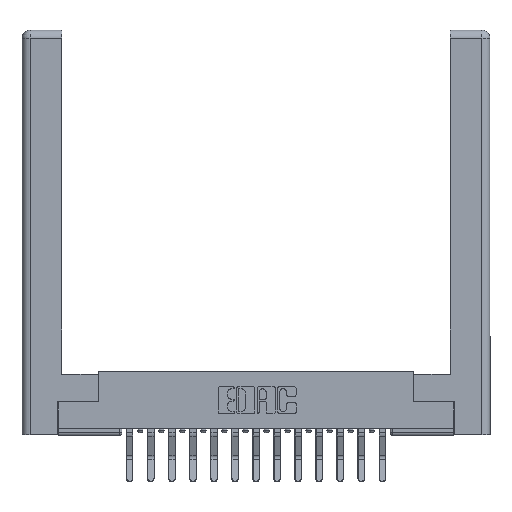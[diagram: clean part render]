
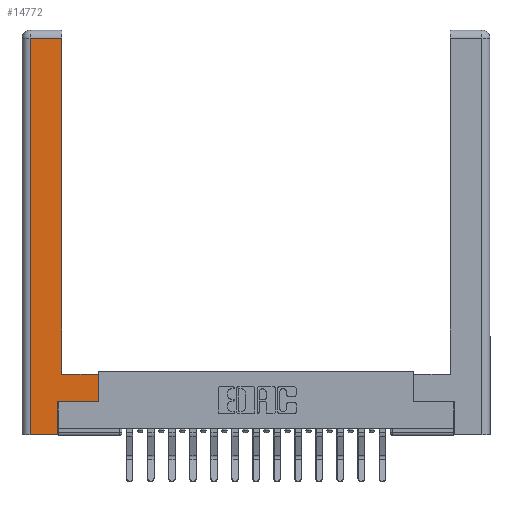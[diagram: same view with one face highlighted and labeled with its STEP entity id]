
A CAD part, top view. The second image highlights one B-rep face of the part: STEP entity #14772.
In plain terms, the highlighted planar face has unit normal (0, 0, 1).
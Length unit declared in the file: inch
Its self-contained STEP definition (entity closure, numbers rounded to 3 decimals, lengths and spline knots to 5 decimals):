
#153 = VECTOR ( 'NONE', #13332, 39.37008 ) ;
#187 = VERTEX_POINT ( 'NONE', #190 ) ;
#190 = CARTESIAN_POINT ( 'NONE',  ( 0.565, 0.245, 0. ) ) ;
#426 = DIRECTION ( 'NONE',  ( 0., 0., -1. ) ) ;
#797 = EDGE_LOOP ( 'NONE', ( #3934, #11235, #12973, #6935, #10437, #15343, #7932, #13033 ) ) ;
#1330 = DIRECTION ( 'NONE',  ( 1., 0., 0. ) ) ;
#1382 = LINE ( 'NONE', #16580, #14872 ) ;
#1908 = VECTOR ( 'NONE', #8428, 39.37008 ) ;
#1924 = VECTOR ( 'NONE', #4143, 39.37008 ) ;
#2317 = VERTEX_POINT ( 'NONE', #4496 ) ;
#2909 = CARTESIAN_POINT ( 'NONE',  ( 0.0615, 2.94, 0. ) ) ;
#2956 = EDGE_CURVE ( 'NONE', #187, #5258, #7629, .T. ) ;
#3008 = CARTESIAN_POINT ( 'NONE',  ( 0.565, 0.245, 0. ) ) ;
#3301 = EDGE_CURVE ( 'NONE', #8868, #14554, #16667, .T. ) ;
#3358 = EDGE_CURVE ( 'NONE', #13544, #8868, #1382, .T. ) ;
#3828 = CARTESIAN_POINT ( 'NONE',  ( 0.265, 0.245, 0. ) ) ;
#3934 = ORIENTED_EDGE ( 'NONE', *, *, #3358, .T. ) ;
#4034 = VECTOR ( 'NONE', #10311, 39.37008 ) ;
#4089 = VERTEX_POINT ( 'NONE', #16123 ) ;
#4143 = DIRECTION ( 'NONE',  ( 0., -1., 0. ) ) ;
#4176 = DIRECTION ( 'NONE',  ( 1., 0., 0. ) ) ;
#4496 = CARTESIAN_POINT ( 'NONE',  ( 0.0615, 0., 0. ) ) ;
#5122 = EDGE_CURVE ( 'NONE', #5258, #13544, #15570, .T. ) ;
#5258 = VERTEX_POINT ( 'NONE', #9324 ) ;
#5654 = LINE ( 'NONE', #17803, #12512 ) ;
#6290 = CARTESIAN_POINT ( 'NONE',  ( 0.295, 0.45, 0. ) ) ;
#6687 = VECTOR ( 'NONE', #10426, 39.37008 ) ;
#6935 = ORIENTED_EDGE ( 'NONE', *, *, #9998, .T. ) ;
#7108 = DIRECTION ( 'NONE',  ( -1., 0., 0. ) ) ;
#7629 = LINE ( 'NONE', #14586, #153 ) ;
#7859 = EDGE_CURVE ( 'NONE', #11265, #4089, #13507, .T. ) ;
#7932 = ORIENTED_EDGE ( 'NONE', *, *, #2956, .T. ) ;
#8428 = DIRECTION ( 'NONE',  ( -1., 0., 0. ) ) ;
#8730 = EDGE_CURVE ( 'NONE', #4089, #187, #11395, .T. ) ;
#8868 = VERTEX_POINT ( 'NONE', #11855 ) ;
#9324 = CARTESIAN_POINT ( 'NONE',  ( 0.565, 0.45, 0. ) ) ;
#9807 = CARTESIAN_POINT ( 'NONE',  ( 0., 0., 0. ) ) ;
#9998 = EDGE_CURVE ( 'NONE', #2317, #11265, #5654, .T. ) ;
#10311 = DIRECTION ( 'NONE',  ( -1., 0., 0. ) ) ;
#10426 = DIRECTION ( 'NONE',  ( 0., 1., 0. ) ) ;
#10437 = ORIENTED_EDGE ( 'NONE', *, *, #7859, .T. ) ;
#11059 = FACE_OUTER_BOUND ( 'NONE', #797, .T. ) ;
#11235 = ORIENTED_EDGE ( 'NONE', *, *, #3301, .T. ) ;
#11265 = VERTEX_POINT ( 'NONE', #14806 ) ;
#11395 = LINE ( 'NONE', #3008, #16839 ) ;
#11855 = CARTESIAN_POINT ( 'NONE',  ( 0.295, 2.94, 0. ) ) ;
#12023 = AXIS2_PLACEMENT_3D ( 'NONE', #9807, #426, #7108 ) ;
#12512 = VECTOR ( 'NONE', #1330, 39.37008 ) ;
#12689 = EDGE_CURVE ( 'NONE', #14554, #2317, #16370, .T. ) ;
#12973 = ORIENTED_EDGE ( 'NONE', *, *, #12689, .T. ) ;
#13033 = ORIENTED_EDGE ( 'NONE', *, *, #5122, .T. ) ;
#13332 = DIRECTION ( 'NONE',  ( 0., 1., 0. ) ) ;
#13507 = LINE ( 'NONE', #3828, #6687 ) ;
#13544 = VERTEX_POINT ( 'NONE', #6290 ) ;
#14554 = VERTEX_POINT ( 'NONE', #17897 ) ;
#14586 = CARTESIAN_POINT ( 'NONE',  ( 0.565, 0.45, 0. ) ) ;
#14772 = ADVANCED_FACE ( 'NONE', ( #11059 ), #16713, .F. ) ;
#14806 = CARTESIAN_POINT ( 'NONE',  ( 0.265, 0., 0. ) ) ;
#14813 = DIRECTION ( 'NONE',  ( 0., 1., 0. ) ) ;
#14872 = VECTOR ( 'NONE', #14813, 39.37008 ) ;
#15343 = ORIENTED_EDGE ( 'NONE', *, *, #8730, .T. ) ;
#15570 = LINE ( 'NONE', #17407, #4034 ) ;
#16123 = CARTESIAN_POINT ( 'NONE',  ( 0.265, 0.245, 0. ) ) ;
#16370 = LINE ( 'NONE', #17828, #1924 ) ;
#16580 = CARTESIAN_POINT ( 'NONE',  ( 0.295, 3., 0. ) ) ;
#16667 = LINE ( 'NONE', #2909, #1908 ) ;
#16713 = PLANE ( 'NONE',  #12023 ) ;
#16839 = VECTOR ( 'NONE', #4176, 39.37008 ) ;
#17407 = CARTESIAN_POINT ( 'NONE',  ( 0.295, 0.45, 0. ) ) ;
#17803 = CARTESIAN_POINT ( 'NONE',  ( 0.265, 0., 0. ) ) ;
#17828 = CARTESIAN_POINT ( 'NONE',  ( 0.0615, 0., 0. ) ) ;
#17897 = CARTESIAN_POINT ( 'NONE',  ( 0.0615, 2.94, 0. ) ) ;
